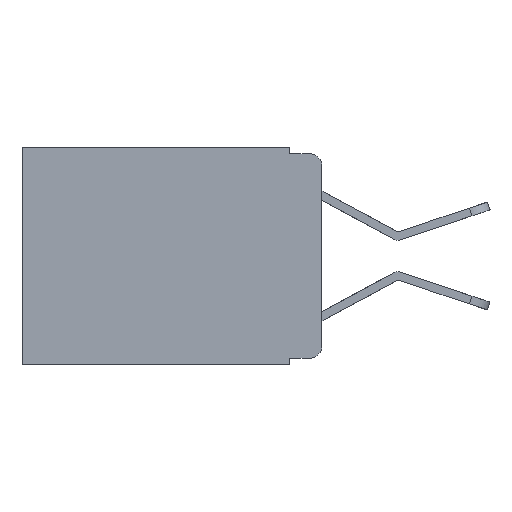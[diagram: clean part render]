
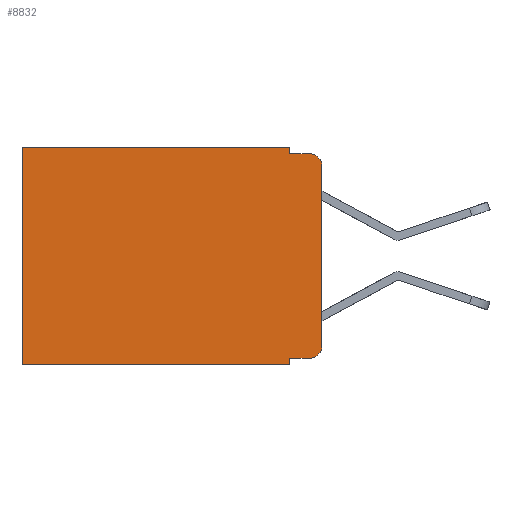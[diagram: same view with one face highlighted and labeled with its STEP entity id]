
A CAD part, left-side view. The second image highlights one B-rep face of the part: STEP entity #8832.
In plain terms, the highlighted planar face has unit normal (-1, 0, 0).
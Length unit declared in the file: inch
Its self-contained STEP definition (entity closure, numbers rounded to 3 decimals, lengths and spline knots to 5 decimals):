
#82 = CIRCLE ( 'NONE', #5084, 0.02 ) ;
#274 = CARTESIAN_POINT ( 'NONE',  ( 0.298, 0., 0. ) ) ;
#328 = CARTESIAN_POINT ( 'NONE',  ( 0.298, 0.02, -0.03 ) ) ;
#584 = CARTESIAN_POINT ( 'NONE',  ( 0.298, 0.051, 0. ) ) ;
#807 = EDGE_CURVE ( 'NONE', #3340, #12076, #5601, .T. ) ;
#913 = LINE ( 'NONE', #10862, #8804 ) ;
#1924 = CARTESIAN_POINT ( 'NONE',  ( 0.298, 0., -0.03 ) ) ;
#1994 = EDGE_CURVE ( 'NONE', #5798, #3650, #11952, .T. ) ;
#2067 = VERTEX_POINT ( 'NONE', #13285 ) ;
#2112 = DIRECTION ( 'NONE',  ( 0., 0., -1. ) ) ;
#2526 = ORIENTED_EDGE ( 'NONE', *, *, #6180, .F. ) ;
#2539 = CARTESIAN_POINT ( 'NONE',  ( 0.298, 0.02, -0.313 ) ) ;
#2582 = CARTESIAN_POINT ( 'NONE',  ( 0.298, 0.051, -0.343 ) ) ;
#2831 = EDGE_LOOP ( 'NONE', ( #2526, #4491, #5944, #14337, #16132, #14135, #19238, #4509, #16810, #15253 ) ) ;
#3032 = EDGE_CURVE ( 'NONE', #3650, #9460, #11447, .T. ) ;
#3340 = VERTEX_POINT ( 'NONE', #9438 ) ;
#3625 = PLANE ( 'NONE',  #18936 ) ;
#3650 = VERTEX_POINT ( 'NONE', #5739 ) ;
#4077 = EDGE_CURVE ( 'NONE', #15917, #9460, #82, .T. ) ;
#4089 = DIRECTION ( 'NONE',  ( 0., 0., -1. ) ) ;
#4199 = CARTESIAN_POINT ( 'NONE',  ( 0.298, 0.473, 0. ) ) ;
#4385 = LINE ( 'NONE', #4503, #16254 ) ;
#4491 = ORIENTED_EDGE ( 'NONE', *, *, #4077, .T. ) ;
#4503 = CARTESIAN_POINT ( 'NONE',  ( 0.298, 0., 0. ) ) ;
#4509 = ORIENTED_EDGE ( 'NONE', *, *, #14519, .F. ) ;
#4561 = FACE_OUTER_BOUND ( 'NONE', #2831, .T. ) ;
#4578 = CARTESIAN_POINT ( 'NONE',  ( 0.298, 0.051, -0.01 ) ) ;
#4708 = VECTOR ( 'NONE', #14088, 39.37008 ) ;
#5084 = AXIS2_PLACEMENT_3D ( 'NONE', #328, #11298, #2112 ) ;
#5237 = VECTOR ( 'NONE', #7879, 39.37008 ) ;
#5601 = LINE ( 'NONE', #4199, #6103 ) ;
#5739 = CARTESIAN_POINT ( 'NONE',  ( 0.298, 0.051, -0.01 ) ) ;
#5798 = VERTEX_POINT ( 'NONE', #15667 ) ;
#5944 = ORIENTED_EDGE ( 'NONE', *, *, #3032, .F. ) ;
#6103 = VECTOR ( 'NONE', #13585, 39.37008 ) ;
#6180 = EDGE_CURVE ( 'NONE', #15917, #2067, #4385, .T. ) ;
#6421 = VERTEX_POINT ( 'NONE', #12895 ) ;
#6789 = DIRECTION ( 'NONE',  ( 0., -1., 0. ) ) ;
#7780 = CARTESIAN_POINT ( 'NONE',  ( 0.298, 0.02, -0.01 ) ) ;
#7879 = DIRECTION ( 'NONE',  ( 0., -1., 0. ) ) ;
#7970 = VECTOR ( 'NONE', #18338, 39.37008 ) ;
#8308 = DIRECTION ( 'NONE',  ( 0., 0., -1. ) ) ;
#8791 = AXIS2_PLACEMENT_3D ( 'NONE', #2539, #13178, #4089 ) ;
#8804 = VECTOR ( 'NONE', #9423, 39.37008 ) ;
#8832 = ADVANCED_FACE ( 'NONE', ( #4561 ), #3625, .F. ) ;
#8860 = LINE ( 'NONE', #16692, #5237 ) ;
#9423 = DIRECTION ( 'NONE',  ( 0., 1., 0. ) ) ;
#9438 = CARTESIAN_POINT ( 'NONE',  ( 0.298, 0.473, 0. ) ) ;
#9460 = VERTEX_POINT ( 'NONE', #7780 ) ;
#10520 = VERTEX_POINT ( 'NONE', #2582 ) ;
#10862 = CARTESIAN_POINT ( 'NONE',  ( 0.298, 0., 0. ) ) ;
#11298 = DIRECTION ( 'NONE',  ( -1., 0., 0. ) ) ;
#11383 = VERTEX_POINT ( 'NONE', #17775 ) ;
#11447 = LINE ( 'NONE', #4578, #11913 ) ;
#11864 = CARTESIAN_POINT ( 'NONE',  ( 0.298, 0.051, 0. ) ) ;
#11913 = VECTOR ( 'NONE', #6789, 39.37008 ) ;
#11952 = LINE ( 'NONE', #11864, #7970 ) ;
#12076 = VERTEX_POINT ( 'NONE', #13409 ) ;
#12621 = EDGE_CURVE ( 'NONE', #11383, #2067, #15752, .T. ) ;
#12662 = CARTESIAN_POINT ( 'NONE',  ( 0.298, 0., -0.343 ) ) ;
#12895 = CARTESIAN_POINT ( 'NONE',  ( 0.298, 0.051, -0.333 ) ) ;
#13178 = DIRECTION ( 'NONE',  ( -1., 0., 0. ) ) ;
#13236 = LINE ( 'NONE', #584, #17002 ) ;
#13285 = CARTESIAN_POINT ( 'NONE',  ( 0.298, 0., -0.313 ) ) ;
#13409 = CARTESIAN_POINT ( 'NONE',  ( 0.298, 0.473, -0.343 ) ) ;
#13579 = EDGE_CURVE ( 'NONE', #6421, #11383, #8860, .T. ) ;
#13585 = DIRECTION ( 'NONE',  ( 0., 0., -1. ) ) ;
#14088 = DIRECTION ( 'NONE',  ( 0., 1., 0. ) ) ;
#14135 = ORIENTED_EDGE ( 'NONE', *, *, #807, .T. ) ;
#14337 = ORIENTED_EDGE ( 'NONE', *, *, #1994, .F. ) ;
#14519 = EDGE_CURVE ( 'NONE', #6421, #10520, #13236, .T. ) ;
#14950 = DIRECTION ( 'NONE',  ( 0., 0., -1. ) ) ;
#15102 = EDGE_CURVE ( 'NONE', #10520, #12076, #16108, .T. ) ;
#15253 = ORIENTED_EDGE ( 'NONE', *, *, #12621, .T. ) ;
#15667 = CARTESIAN_POINT ( 'NONE',  ( 0.298, 0.051, 0. ) ) ;
#15752 = CIRCLE ( 'NONE', #8791, 0.02 ) ;
#15797 = DIRECTION ( 'NONE',  ( 0., 0., -1. ) ) ;
#15815 = EDGE_CURVE ( 'NONE', #5798, #3340, #913, .T. ) ;
#15917 = VERTEX_POINT ( 'NONE', #1924 ) ;
#16108 = LINE ( 'NONE', #12662, #4708 ) ;
#16132 = ORIENTED_EDGE ( 'NONE', *, *, #15815, .T. ) ;
#16254 = VECTOR ( 'NONE', #14950, 39.37008 ) ;
#16692 = CARTESIAN_POINT ( 'NONE',  ( 0.298, 0.051, -0.333 ) ) ;
#16810 = ORIENTED_EDGE ( 'NONE', *, *, #13579, .T. ) ;
#17002 = VECTOR ( 'NONE', #15797, 39.37008 ) ;
#17032 = DIRECTION ( 'NONE',  ( 1., 0., 0. ) ) ;
#17775 = CARTESIAN_POINT ( 'NONE',  ( 0.298, 0.02, -0.333 ) ) ;
#18338 = DIRECTION ( 'NONE',  ( 0., 0., -1. ) ) ;
#18936 = AXIS2_PLACEMENT_3D ( 'NONE', #274, #17032, #8308 ) ;
#19238 = ORIENTED_EDGE ( 'NONE', *, *, #15102, .F. ) ;
